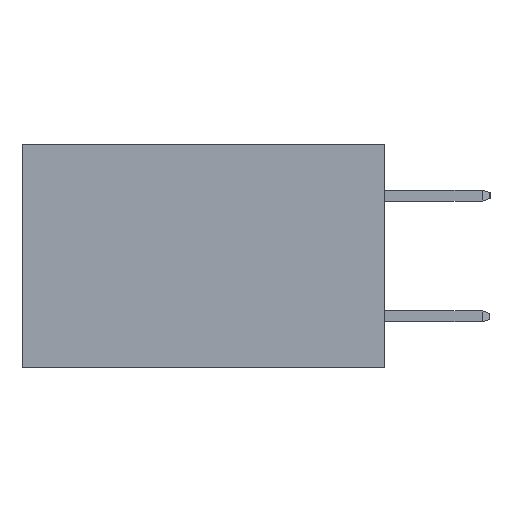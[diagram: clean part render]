
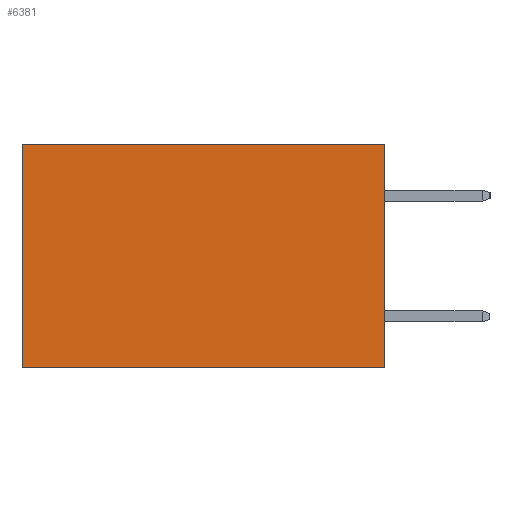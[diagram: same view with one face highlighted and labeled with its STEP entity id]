
A CAD part, left-side view. The second image highlights one B-rep face of the part: STEP entity #6381.
In plain terms, the highlighted planar face has unit normal (-1, 0, 0).
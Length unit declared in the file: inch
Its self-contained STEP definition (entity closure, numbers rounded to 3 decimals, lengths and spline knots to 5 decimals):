
#1087 = VERTEX_POINT ( 'NONE', #3272 ) ;
#1845 = LINE ( 'NONE', #13148, #15318 ) ;
#2276 = VERTEX_POINT ( 'NONE', #15507 ) ;
#2538 = EDGE_CURVE ( 'NONE', #3143, #1087, #2595, .T. ) ;
#2595 = LINE ( 'NONE', #15666, #16006 ) ;
#2968 = CARTESIAN_POINT ( 'NONE',  ( 0.298, 0.6, 0. ) ) ;
#3143 = VERTEX_POINT ( 'NONE', #5342 ) ;
#3272 = CARTESIAN_POINT ( 'NONE',  ( 0.298, 0.6, -0.37 ) ) ;
#4260 = CARTESIAN_POINT ( 'NONE',  ( 0.298, 0., 0. ) ) ;
#4284 = AXIS2_PLACEMENT_3D ( 'NONE', #16514, #16236, #16180 ) ;
#4302 = DIRECTION ( 'NONE',  ( 0., 1., 0. ) ) ;
#5092 = ORIENTED_EDGE ( 'NONE', *, *, #12849, .T. ) ;
#5342 = CARTESIAN_POINT ( 'NONE',  ( 0.298, 0., -0.37 ) ) ;
#5670 = ORIENTED_EDGE ( 'NONE', *, *, #2538, .F. ) ;
#6247 = EDGE_CURVE ( 'NONE', #14018, #3143, #1845, .T. ) ;
#6381 = ADVANCED_FACE ( 'NONE', ( #7271 ), #16285, .F. ) ;
#7271 = FACE_OUTER_BOUND ( 'NONE', #15627, .T. ) ;
#7588 = ORIENTED_EDGE ( 'NONE', *, *, #6247, .F. ) ;
#8257 = LINE ( 'NONE', #4260, #14726 ) ;
#8398 = ORIENTED_EDGE ( 'NONE', *, *, #12120, .T. ) ;
#8708 = DIRECTION ( 'NONE',  ( 0., 0., -1. ) ) ;
#9299 = CARTESIAN_POINT ( 'NONE',  ( 0.298, 0., 0. ) ) ;
#10865 = DIRECTION ( 'NONE',  ( 0., 0., -1. ) ) ;
#10866 = VECTOR ( 'NONE', #10865, 39.37008 ) ;
#12120 = EDGE_CURVE ( 'NONE', #14018, #2276, #8257, .T. ) ;
#12849 = EDGE_CURVE ( 'NONE', #2276, #1087, #13912, .T. ) ;
#13148 = CARTESIAN_POINT ( 'NONE',  ( 0.298, 0., 0. ) ) ;
#13912 = LINE ( 'NONE', #2968, #10866 ) ;
#14018 = VERTEX_POINT ( 'NONE', #9299 ) ;
#14726 = VECTOR ( 'NONE', #4302, 39.37008 ) ;
#15318 = VECTOR ( 'NONE', #8708, 39.37008 ) ;
#15507 = CARTESIAN_POINT ( 'NONE',  ( 0.298, 0.6, 0. ) ) ;
#15627 = EDGE_LOOP ( 'NONE', ( #5092, #5670, #7588, #8398 ) ) ;
#15654 = DIRECTION ( 'NONE',  ( 0., 1., 0. ) ) ;
#15666 = CARTESIAN_POINT ( 'NONE',  ( 0.298, 0., -0.37 ) ) ;
#16006 = VECTOR ( 'NONE', #15654, 39.37008 ) ;
#16180 = DIRECTION ( 'NONE',  ( 0., 0., -1. ) ) ;
#16236 = DIRECTION ( 'NONE',  ( 1., 0., 0. ) ) ;
#16285 = PLANE ( 'NONE',  #4284 ) ;
#16514 = CARTESIAN_POINT ( 'NONE',  ( 0.298, 0., 0. ) ) ;
